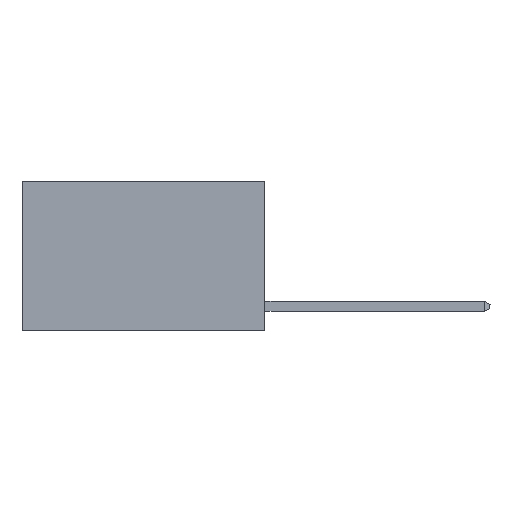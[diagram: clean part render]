
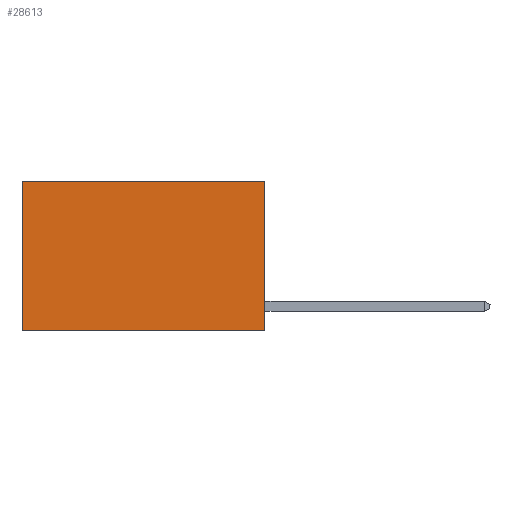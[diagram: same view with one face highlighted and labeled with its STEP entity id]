
A CAD part, left-side view. The second image highlights one B-rep face of the part: STEP entity #28613.
In plain terms, the highlighted planar face has unit normal (-1, 0, 0).
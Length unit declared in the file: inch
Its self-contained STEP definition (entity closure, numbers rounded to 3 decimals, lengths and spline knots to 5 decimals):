
#700 = ORIENTED_EDGE ( 'NONE', *, *, #28467, .F. ) ;
#892 = EDGE_CURVE ( 'NONE', #21035, #16637, #13946, .T. ) ;
#3892 = DIRECTION ( 'NONE',  ( 0., 1., 0. ) ) ;
#4367 = LINE ( 'NONE', #18215, #7233 ) ;
#5316 = VERTEX_POINT ( 'NONE', #7885 ) ;
#7233 = VECTOR ( 'NONE', #8753, 39.37008 ) ;
#7885 = CARTESIAN_POINT ( 'NONE',  ( 0.2625, 0.6, -0.37 ) ) ;
#8753 = DIRECTION ( 'NONE',  ( 0., 0., -1. ) ) ;
#9146 = DIRECTION ( 'NONE',  ( 1., 0., 0. ) ) ;
#9157 = CARTESIAN_POINT ( 'NONE',  ( 0.2625, 0.6, 0. ) ) ;
#11118 = FACE_OUTER_BOUND ( 'NONE', #18785, .T. ) ;
#11651 = AXIS2_PLACEMENT_3D ( 'NONE', #22983, #9146, #29456 ) ;
#13076 = CARTESIAN_POINT ( 'NONE',  ( 0.2625, 0., -0.37 ) ) ;
#13139 = VECTOR ( 'NONE', #25657, 39.37008 ) ;
#13946 = LINE ( 'NONE', #14246, #13139 ) ;
#14246 = CARTESIAN_POINT ( 'NONE',  ( 0.2625, 0., 0. ) ) ;
#15581 = ORIENTED_EDGE ( 'NONE', *, *, #28955, .T. ) ;
#16637 = VERTEX_POINT ( 'NONE', #9157 ) ;
#17989 = CARTESIAN_POINT ( 'NONE',  ( 0.2625, 0.6, 0. ) ) ;
#18215 = CARTESIAN_POINT ( 'NONE',  ( 0.2625, 0., 0. ) ) ;
#18785 = EDGE_LOOP ( 'NONE', ( #15581, #700, #24445, #22003 ) ) ;
#18886 = VECTOR ( 'NONE', #29562, 39.37008 ) ;
#20135 = LINE ( 'NONE', #13076, #25101 ) ;
#20573 = PLANE ( 'NONE',  #11651 ) ;
#21035 = VERTEX_POINT ( 'NONE', #29315 ) ;
#22003 = ORIENTED_EDGE ( 'NONE', *, *, #892, .T. ) ;
#22983 = CARTESIAN_POINT ( 'NONE',  ( 0.2625, 0., 0. ) ) ;
#24437 = EDGE_CURVE ( 'NONE', #21035, #27422, #4367, .T. ) ;
#24445 = ORIENTED_EDGE ( 'NONE', *, *, #24437, .F. ) ;
#25101 = VECTOR ( 'NONE', #3892, 39.37008 ) ;
#25657 = DIRECTION ( 'NONE',  ( 0., 1., 0. ) ) ;
#27422 = VERTEX_POINT ( 'NONE', #29367 ) ;
#28467 = EDGE_CURVE ( 'NONE', #27422, #5316, #20135, .T. ) ;
#28613 = ADVANCED_FACE ( 'NONE', ( #11118 ), #20573, .F. ) ;
#28955 = EDGE_CURVE ( 'NONE', #16637, #5316, #29707, .T. ) ;
#29315 = CARTESIAN_POINT ( 'NONE',  ( 0.2625, 0., 0. ) ) ;
#29367 = CARTESIAN_POINT ( 'NONE',  ( 0.2625, 0., -0.37 ) ) ;
#29456 = DIRECTION ( 'NONE',  ( 0., 0., -1. ) ) ;
#29562 = DIRECTION ( 'NONE',  ( 0., 0., -1. ) ) ;
#29707 = LINE ( 'NONE', #17989, #18886 ) ;
